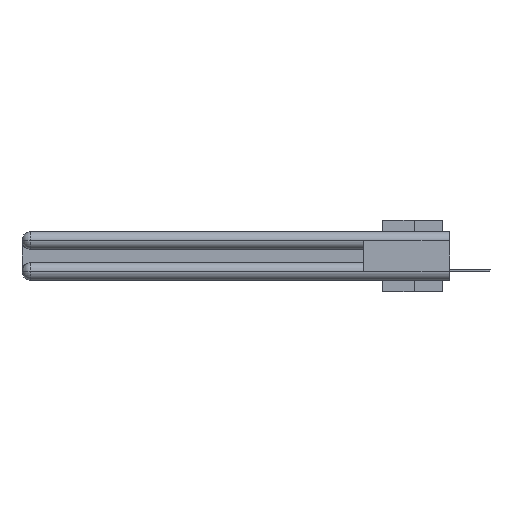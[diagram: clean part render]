
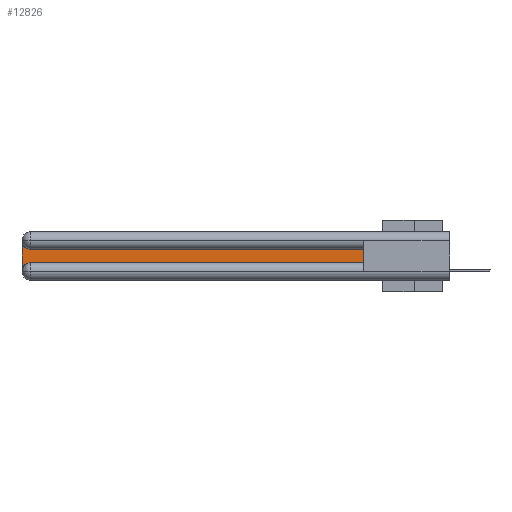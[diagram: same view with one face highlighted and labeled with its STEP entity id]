
A CAD part, left-side view. The second image highlights one B-rep face of the part: STEP entity #12826.
In plain terms, the highlighted planar face has unit normal (-1, 0, 0).
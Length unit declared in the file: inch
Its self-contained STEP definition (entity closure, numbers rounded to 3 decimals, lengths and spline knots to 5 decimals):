
#106 = VERTEX_POINT ( 'NONE', #9583 ) ;
#443 = DIRECTION ( 'NONE',  ( 0., 0., -1. ) ) ;
#697 = DIRECTION ( 'NONE',  ( 0., 0., -1. ) ) ;
#1059 = DIRECTION ( 'NONE',  ( 1., 0., 0. ) ) ;
#1083 = ORIENTED_EDGE ( 'NONE', *, *, #21722, .T. ) ;
#2178 = EDGE_LOOP ( 'NONE', ( #24204, #11591, #1083, #24664, #19517, #14469 ) ) ;
#2823 = DIRECTION ( 'NONE',  ( 1., 0., 0. ) ) ;
#3864 = CARTESIAN_POINT ( 'NONE',  ( 0.075, 0.6, -0.2175 ) ) ;
#4608 = EDGE_CURVE ( 'NONE', #21530, #5626, #5997, .T. ) ;
#4928 = CARTESIAN_POINT ( 'NONE',  ( 0.075, 2.94, -0.1225 ) ) ;
#5626 = VERTEX_POINT ( 'NONE', #23682 ) ;
#5997 = LINE ( 'NONE', #13261, #23164 ) ;
#6404 = VERTEX_POINT ( 'NONE', #10314 ) ;
#6933 = VECTOR ( 'NONE', #10428, 39.37008 ) ;
#7013 = AXIS2_PLACEMENT_3D ( 'NONE', #26315, #2823, #12243 ) ;
#7287 = PLANE ( 'NONE',  #7013 ) ;
#8473 = LINE ( 'NONE', #20241, #20771 ) ;
#8896 = VERTEX_POINT ( 'NONE', #25704 ) ;
#9189 = VECTOR ( 'NONE', #25032, 39.37008 ) ;
#9583 = CARTESIAN_POINT ( 'NONE',  ( 0.075, 3., -0.0625 ) ) ;
#9751 = FACE_OUTER_BOUND ( 'NONE', #2178, .T. ) ;
#9879 = EDGE_CURVE ( 'NONE', #27411, #106, #27895, .T. ) ;
#10314 = CARTESIAN_POINT ( 'NONE',  ( 0.075, 2.94, -0.2175 ) ) ;
#10428 = DIRECTION ( 'NONE',  ( 0., 0., -1. ) ) ;
#10936 = DIRECTION ( 'NONE',  ( 0., 0., 1. ) ) ;
#11036 = LINE ( 'NONE', #22186, #6933 ) ;
#11591 = ORIENTED_EDGE ( 'NONE', *, *, #9879, .T. ) ;
#12243 = DIRECTION ( 'NONE',  ( 0., 0., -1. ) ) ;
#12826 = ADVANCED_FACE ( 'NONE', ( #9751 ), #7287, .F. ) ;
#13120 = LINE ( 'NONE', #27350, #9189 ) ;
#13261 = CARTESIAN_POINT ( 'NONE',  ( 0.075, 0.6, -0.2175 ) ) ;
#13589 = DIRECTION ( 'NONE',  ( 0., -1., 0. ) ) ;
#14469 = ORIENTED_EDGE ( 'NONE', *, *, #4608, .T. ) ;
#15944 = EDGE_CURVE ( 'NONE', #8896, #6404, #23949, .T. ) ;
#18574 = EDGE_CURVE ( 'NONE', #5626, #27411, #13120, .T. ) ;
#19517 = ORIENTED_EDGE ( 'NONE', *, *, #21414, .T. ) ;
#19693 = CARTESIAN_POINT ( 'NONE',  ( 0.075, 2.94, -0.0625 ) ) ;
#20241 = CARTESIAN_POINT ( 'NONE',  ( 0.075, 0.6, -0.2175 ) ) ;
#20771 = VECTOR ( 'NONE', #13589, 39.37008 ) ;
#21414 = EDGE_CURVE ( 'NONE', #6404, #21530, #8473, .T. ) ;
#21530 = VERTEX_POINT ( 'NONE', #3864 ) ;
#21722 = EDGE_CURVE ( 'NONE', #106, #8896, #11036, .T. ) ;
#22186 = CARTESIAN_POINT ( 'NONE',  ( 0.075, 3., -0.2175 ) ) ;
#23164 = VECTOR ( 'NONE', #10936, 39.37008 ) ;
#23682 = CARTESIAN_POINT ( 'NONE',  ( 0.075, 0.6, -0.1225 ) ) ;
#23949 = CIRCLE ( 'NONE', #29383, 0.06 ) ;
#24204 = ORIENTED_EDGE ( 'NONE', *, *, #18574, .T. ) ;
#24664 = ORIENTED_EDGE ( 'NONE', *, *, #15944, .T. ) ;
#25032 = DIRECTION ( 'NONE',  ( 0., 1., 0. ) ) ;
#25704 = CARTESIAN_POINT ( 'NONE',  ( 0.075, 3., -0.2775 ) ) ;
#26315 = CARTESIAN_POINT ( 'NONE',  ( 0.075, 3., -0.1225 ) ) ;
#26415 = AXIS2_PLACEMENT_3D ( 'NONE', #19693, #29129, #697 ) ;
#27350 = CARTESIAN_POINT ( 'NONE',  ( 0.075, 0.6, -0.1225 ) ) ;
#27411 = VERTEX_POINT ( 'NONE', #4928 ) ;
#27895 = CIRCLE ( 'NONE', #26415, 0.06 ) ;
#29030 = CARTESIAN_POINT ( 'NONE',  ( 0.075, 2.94, -0.2775 ) ) ;
#29129 = DIRECTION ( 'NONE',  ( 1., 0., 0. ) ) ;
#29383 = AXIS2_PLACEMENT_3D ( 'NONE', #29030, #1059, #443 ) ;
